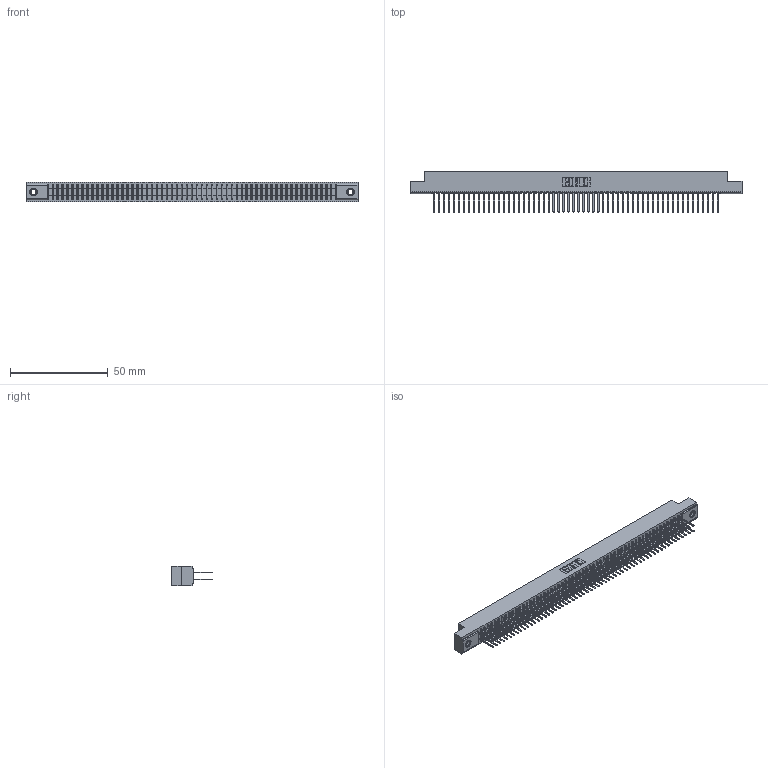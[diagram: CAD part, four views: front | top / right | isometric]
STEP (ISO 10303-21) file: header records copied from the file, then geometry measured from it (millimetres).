
FILE_DESCRIPTION (( 'STEP AP203' ), '1' );
FILE_NAME ('341-116-522-207.STEP', '2018-08-08T13:59:21', ( '' ), ( '' ), 'SwSTEP 2.0', 'SolidWorks 2016', '' );
FILE_SCHEMA (( 'CONFIG_CONTROL_DESIGN' ));
Length unit declared in the file: inch
Products named in the file (4): 341-116-522-207; 341 Part_.156 (3.96) Dia Mounting Holes; 341-292-001_341-292-122; 345-250-001_345-250-005-103
Assembly tree (119 placements, depth 2):
  341-116-522-207
    341 Part_.156 (3.96) Dia Mounting Holes
    341-292-001_341-292-122  x116
    345-250-001_345-250-005-103  x2
Bounding box: 169.54 x 20.62 x 10.16 mm (x, y, z)
Volume: 12679.6 mm3; surface area: 24087.1 mm2
Topology: 119 solids, 119 shells, 7832 faces, 22666 edges, 14674 vertices
Faces by surface type: plane 4740, cylinder 2844, sphere 118, torus 118, cone 12
Entity records: 69246 total; most frequent: CARTESIAN_POINT 11493, ORIENTED_EDGE 11416, DIRECTION 11152, EDGE_CURVE 5708, LINE 4626, VECTOR 4626, VERTEX_POINT 3604, AXIS2_PLACEMENT_3D 3263
